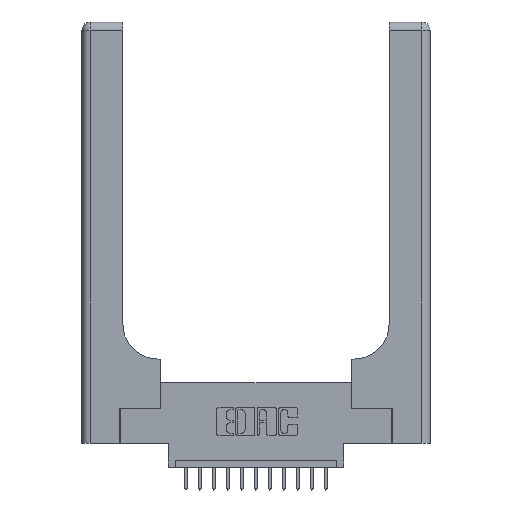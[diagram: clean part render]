
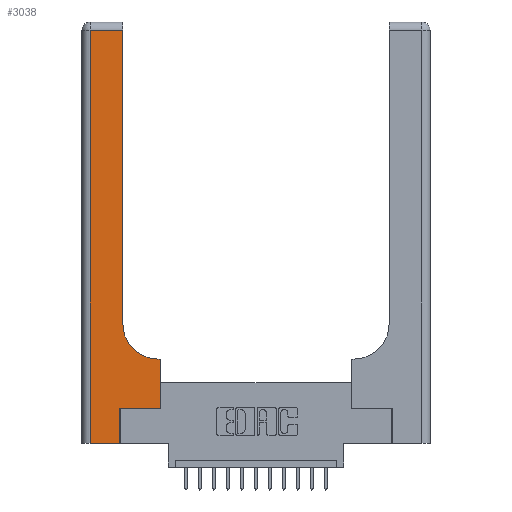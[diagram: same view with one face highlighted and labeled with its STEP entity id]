
A CAD part, top view. The second image highlights one B-rep face of the part: STEP entity #3038.
In plain terms, the highlighted planar face has unit normal (0, 0, 1).
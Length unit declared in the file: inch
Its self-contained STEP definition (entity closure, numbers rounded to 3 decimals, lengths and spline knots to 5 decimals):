
#50 = CARTESIAN_POINT ( 'NONE',  ( 0.5585, 0.6, 0.37 ) ) ;
#59 = CARTESIAN_POINT ( 'NONE',  ( 0.5415, 0.85, 0.37 ) ) ;
#477 = PLANE ( 'NONE',  #17317 ) ;
#1086 = LINE ( 'NONE', #6667, #12261 ) ;
#1314 = CARTESIAN_POINT ( 'NONE',  ( 0.269, 0.25, 0.37 ) ) ;
#1403 = ORIENTED_EDGE ( 'NONE', *, *, #3215, .T. ) ;
#1871 = CARTESIAN_POINT ( 'NONE',  ( 0.06, 0., 0.37 ) ) ;
#2257 = ORIENTED_EDGE ( 'NONE', *, *, #14618, .T. ) ;
#2493 = VERTEX_POINT ( 'NONE', #50 ) ;
#2532 = DIRECTION ( 'NONE',  ( -1., 0., 0. ) ) ;
#2669 = VECTOR ( 'NONE', #8686, 39.37008 ) ;
#2738 = VECTOR ( 'NONE', #2532, 39.37008 ) ;
#2819 = DIRECTION ( 'NONE',  ( 1., 0., 0. ) ) ;
#2839 = DIRECTION ( 'NONE',  ( 0., 1., 0. ) ) ;
#3038 = ADVANCED_FACE ( 'NONE', ( #13488 ), #477, .F. ) ;
#3161 = LINE ( 'NONE', #3716, #6397 ) ;
#3196 = ORIENTED_EDGE ( 'NONE', *, *, #3235, .T. ) ;
#3215 = EDGE_CURVE ( 'NONE', #15721, #12705, #3161, .T. ) ;
#3235 = EDGE_CURVE ( 'NONE', #11161, #15721, #14587, .T. ) ;
#3239 = VERTEX_POINT ( 'NONE', #12034 ) ;
#3417 = DIRECTION ( 'NONE',  ( 0., 0., -1. ) ) ;
#3461 = VERTEX_POINT ( 'NONE', #16846 ) ;
#3716 = CARTESIAN_POINT ( 'NONE',  ( 0.06, 3., 0.37 ) ) ;
#4436 = VECTOR ( 'NONE', #2819, 39.37008 ) ;
#4478 = VECTOR ( 'NONE', #15996, 39.37008 ) ;
#4679 = LINE ( 'NONE', #7036, #5125 ) ;
#5125 = VECTOR ( 'NONE', #2839, 39.37008 ) ;
#5241 = EDGE_CURVE ( 'NONE', #2493, #9991, #10880, .T. ) ;
#5771 = VECTOR ( 'NONE', #17797, 39.37008 ) ;
#6062 = AXIS2_PLACEMENT_3D ( 'NONE', #59, #17830, #10972 ) ;
#6128 = ORIENTED_EDGE ( 'NONE', *, *, #8339, .T. ) ;
#6397 = VECTOR ( 'NONE', #10621, 39.37008 ) ;
#6507 = CARTESIAN_POINT ( 'NONE',  ( 0.2915, 2.94, 0.37 ) ) ;
#6587 = CARTESIAN_POINT ( 'NONE',  ( 0.5585, 0.25, 0.37 ) ) ;
#6667 = CARTESIAN_POINT ( 'NONE',  ( 0.2915, 3., 0.37 ) ) ;
#6911 = CARTESIAN_POINT ( 'NONE',  ( 0.2915, 0.85, 0.37 ) ) ;
#7036 = CARTESIAN_POINT ( 'NONE',  ( 0.269, 0., 0.37 ) ) ;
#7720 = EDGE_CURVE ( 'NONE', #17060, #11161, #1086, .T. ) ;
#7889 = ORIENTED_EDGE ( 'NONE', *, *, #7720, .T. ) ;
#8013 = CARTESIAN_POINT ( 'NONE',  ( 0., 2.94, 0.37 ) ) ;
#8339 = EDGE_CURVE ( 'NONE', #3461, #2493, #16778, .T. ) ;
#8686 = DIRECTION ( 'NONE',  ( -1., 0., 0. ) ) ;
#9088 = CARTESIAN_POINT ( 'NONE',  ( 0., 0., 0.37 ) ) ;
#9675 = VERTEX_POINT ( 'NONE', #11584 ) ;
#9991 = VERTEX_POINT ( 'NONE', #17312 ) ;
#10291 = LINE ( 'NONE', #1314, #4436 ) ;
#10621 = DIRECTION ( 'NONE',  ( 0., -1., 0. ) ) ;
#10667 = CARTESIAN_POINT ( 'NONE',  ( 0.06, 2.94, 0.37 ) ) ;
#10824 = ORIENTED_EDGE ( 'NONE', *, *, #14169, .T. ) ;
#10859 = ORIENTED_EDGE ( 'NONE', *, *, #13381, .T. ) ;
#10880 = LINE ( 'NONE', #11457, #2669 ) ;
#10972 = DIRECTION ( 'NONE',  ( 1., 0., 0. ) ) ;
#11161 = VERTEX_POINT ( 'NONE', #6507 ) ;
#11457 = CARTESIAN_POINT ( 'NONE',  ( 0.2915, 0.6, 0.37 ) ) ;
#11584 = CARTESIAN_POINT ( 'NONE',  ( 0.269, 0., 0.37 ) ) ;
#12034 = CARTESIAN_POINT ( 'NONE',  ( 0.269, 0.25, 0.37 ) ) ;
#12070 = ORIENTED_EDGE ( 'NONE', *, *, #5241, .T. ) ;
#12261 = VECTOR ( 'NONE', #16464, 39.37008 ) ;
#12705 = VERTEX_POINT ( 'NONE', #1871 ) ;
#12777 = CARTESIAN_POINT ( 'NONE',  ( 0., 3., 0.37 ) ) ;
#12885 = EDGE_LOOP ( 'NONE', ( #7889, #3196, #1403, #10859, #10824, #16570, #6128, #12070, #2257 ) ) ;
#12905 = DIRECTION ( 'NONE',  ( -1., 0., 0. ) ) ;
#13093 = LINE ( 'NONE', #9088, #4478 ) ;
#13381 = EDGE_CURVE ( 'NONE', #12705, #9675, #13093, .T. ) ;
#13488 = FACE_OUTER_BOUND ( 'NONE', #12885, .T. ) ;
#13905 = CIRCLE ( 'NONE', #6062, 0.25 ) ;
#14169 = EDGE_CURVE ( 'NONE', #9675, #3239, #4679, .T. ) ;
#14587 = LINE ( 'NONE', #8013, #2738 ) ;
#14618 = EDGE_CURVE ( 'NONE', #9991, #17060, #13905, .T. ) ;
#14668 = EDGE_CURVE ( 'NONE', #3239, #3461, #10291, .T. ) ;
#15721 = VERTEX_POINT ( 'NONE', #10667 ) ;
#15996 = DIRECTION ( 'NONE',  ( 1., 0., 0. ) ) ;
#16464 = DIRECTION ( 'NONE',  ( 0., 1., 0. ) ) ;
#16570 = ORIENTED_EDGE ( 'NONE', *, *, #14668, .T. ) ;
#16778 = LINE ( 'NONE', #6587, #5771 ) ;
#16846 = CARTESIAN_POINT ( 'NONE',  ( 0.5585, 0.25, 0.37 ) ) ;
#17060 = VERTEX_POINT ( 'NONE', #6911 ) ;
#17312 = CARTESIAN_POINT ( 'NONE',  ( 0.5415, 0.6, 0.37 ) ) ;
#17317 = AXIS2_PLACEMENT_3D ( 'NONE', #12777, #3417, #12905 ) ;
#17797 = DIRECTION ( 'NONE',  ( 0., 1., 0. ) ) ;
#17830 = DIRECTION ( 'NONE',  ( 0., 0., -1. ) ) ;
